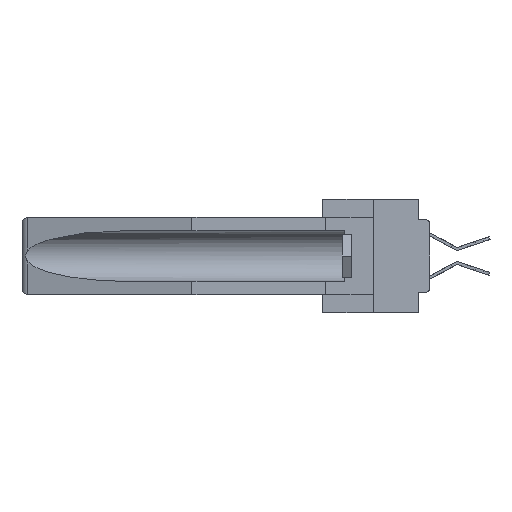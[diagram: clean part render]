
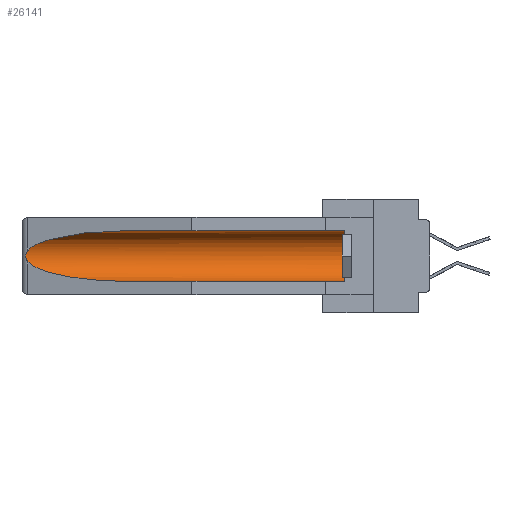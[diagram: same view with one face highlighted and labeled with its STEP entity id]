
A CAD part, left-side view. The second image highlights one B-rep face of the part: STEP entity #26141.
In plain terms, the highlighted cylindrical face has radius 2.857 mm (diameter 5.715 mm), a partial arc.
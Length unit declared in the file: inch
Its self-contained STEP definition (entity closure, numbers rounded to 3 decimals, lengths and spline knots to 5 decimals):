
#2087 = EDGE_LOOP ( 'NONE', ( #5907, #36978, #5419, #32253, #24840, #16142 ) ) ;
#3208 = CARTESIAN_POINT ( 'NONE',  ( 0.155, 1.07973, -0.059 ) ) ;
#3532 = AXIS2_PLACEMENT_3D ( 'NONE', #27109, #9231, #17881 ) ;
#4815 =( BOUNDED_CURVE ( )  B_SPLINE_CURVE ( 3, ( #15616, #17780, #27006, #27587 ),
 .UNSPECIFIED., .F., .F. ) 
 B_SPLINE_CURVE_WITH_KNOTS ( ( 4, 4 ),
 ( 0.1948, 1.5708 ),
 .UNSPECIFIED. ) 
 CURVE ( )  GEOMETRIC_REPRESENTATION_ITEM ( )  RATIONAL_B_SPLINE_CURVE ( ( 1., 0.848, 0.848, 1. ) ) 
 REPRESENTATION_ITEM ( '' )  );
#5419 = ORIENTED_EDGE ( 'NONE', *, *, #8309, .T. ) ;
#5594 = EDGE_CURVE ( 'NONE', #26791, #5600, #10086, .T. ) ;
#5600 = VERTEX_POINT ( 'NONE', #36031 ) ;
#5656 = CARTESIAN_POINT ( 'NONE',  ( 0.26655, 1.53094, -0.18657 ) ) ;
#5907 = ORIENTED_EDGE ( 'NONE', *, *, #5594, .T. ) ;
#7216 = VECTOR ( 'NONE', #13653, 39.37008 ) ;
#7429 = B_SPLINE_CURVE_WITH_KNOTS ( 'NONE', 3,
 ( #32557, #29431, #37891, #14514, #26503, #23558, #7831, #5656, #17658, #14709 ),
 .UNSPECIFIED., .F., .F.,
 ( 4, 2, 2, 2, 4 ),
 ( 0., 0.00029, 0.00058, 0.00087, 0.00117 ),
 .UNSPECIFIED. ) ;
#7769 = CARTESIAN_POINT ( 'NONE',  ( 0.155, 0.126, -0.059 ) ) ;
#7831 = CARTESIAN_POINT ( 'NONE',  ( 0.2673, 1.53269, -0.17917 ) ) ;
#8309 = EDGE_CURVE ( 'NONE', #30241, #24768, #4815, .T. ) ;
#8331 = VERTEX_POINT ( 'NONE', #15031 ) ;
#9231 = DIRECTION ( 'NONE',  ( 0., -1., 0. ) ) ;
#9416 = CARTESIAN_POINT ( 'NONE',  ( 0.26537, 1.52718, -0.19328 ) ) ;
#10086 =( BOUNDED_CURVE ( )  B_SPLINE_CURVE ( 3, ( #12041, #15400, #24240, #36415 ),
 .UNSPECIFIED., .F., .F. ) 
 B_SPLINE_CURVE_WITH_KNOTS ( ( 4, 4 ),
 ( 4.71239, 6.08839 ),
 .UNSPECIFIED. ) 
 CURVE ( )  GEOMETRIC_REPRESENTATION_ITEM ( )  RATIONAL_B_SPLINE_CURVE ( ( 1., 0.848, 0.848, 1. ) ) 
 REPRESENTATION_ITEM ( '' )  );
#10469 = EDGE_CURVE ( 'NONE', #5600, #30241, #7429, .T. ) ;
#10887 = CARTESIAN_POINT ( 'NONE',  ( 0.155, -0.30754, -0.284 ) ) ;
#12041 = CARTESIAN_POINT ( 'NONE',  ( 0.155, 1.07973, -0.059 ) ) ;
#12515 = DIRECTION ( 'NONE',  ( 0., 0., 1. ) ) ;
#13653 = DIRECTION ( 'NONE',  ( 0., 1., 0. ) ) ;
#14514 = CARTESIAN_POINT ( 'NONE',  ( 0.2673, 1.5327, -0.16383 ) ) ;
#14709 = CARTESIAN_POINT ( 'NONE',  ( 0.26537, 1.52718, -0.19328 ) ) ;
#15031 = CARTESIAN_POINT ( 'NONE',  ( 0.155, 0.126, -0.284 ) ) ;
#15400 = CARTESIAN_POINT ( 'NONE',  ( 0.21114, 1.30732, -0.059 ) ) ;
#15616 = CARTESIAN_POINT ( 'NONE',  ( 0.26537, 1.52718, -0.19328 ) ) ;
#16083 = EDGE_CURVE ( 'NONE', #8331, #24768, #29150, .T. ) ;
#16142 = ORIENTED_EDGE ( 'NONE', *, *, #20110, .T. ) ;
#16235 = LINE ( 'NONE', #25461, #25665 ) ;
#17658 = CARTESIAN_POINT ( 'NONE',  ( 0.26597, 1.5296, -0.19026 ) ) ;
#17780 = CARTESIAN_POINT ( 'NONE',  ( 0.25451, 1.48313, -0.24835 ) ) ;
#17881 = DIRECTION ( 'NONE',  ( 0., 0., 1. ) ) ;
#18233 = CYLINDRICAL_SURFACE ( 'NONE', #36060, 0.1125 ) ;
#19580 = DIRECTION ( 'NONE',  ( 0., 1., 0. ) ) ;
#20110 = EDGE_CURVE ( 'NONE', #21517, #26791, #16235, .T. ) ;
#20983 = DIRECTION ( 'NONE',  ( 0., 1., 0. ) ) ;
#21517 = VERTEX_POINT ( 'NONE', #7769 ) ;
#21754 = FACE_OUTER_BOUND ( 'NONE', #2087, .T. ) ;
#22970 = CIRCLE ( 'NONE', #3532, 0.1125 ) ;
#23558 = CARTESIAN_POINT ( 'NONE',  ( 0.2675, 1.53308, -0.17534 ) ) ;
#24240 = CARTESIAN_POINT ( 'NONE',  ( 0.25451, 1.48313, -0.09465 ) ) ;
#24768 = VERTEX_POINT ( 'NONE', #37865 ) ;
#24840 = ORIENTED_EDGE ( 'NONE', *, *, #36163, .T. ) ;
#25461 = CARTESIAN_POINT ( 'NONE',  ( 0.155, -0.30754, -0.059 ) ) ;
#25665 = VECTOR ( 'NONE', #19580, 39.37008 ) ;
#26141 = ADVANCED_FACE ( 'NONE', ( #21754 ), #18233, .F. ) ;
#26503 = CARTESIAN_POINT ( 'NONE',  ( 0.2675, 1.53308, -0.16763 ) ) ;
#26791 = VERTEX_POINT ( 'NONE', #3208 ) ;
#27006 = CARTESIAN_POINT ( 'NONE',  ( 0.21114, 1.30732, -0.284 ) ) ;
#27109 = CARTESIAN_POINT ( 'NONE',  ( 0.155, 0.126, -0.1715 ) ) ;
#27587 = CARTESIAN_POINT ( 'NONE',  ( 0.155, 1.07973, -0.284 ) ) ;
#29150 = LINE ( 'NONE', #10887, #7216 ) ;
#29431 = CARTESIAN_POINT ( 'NONE',  ( 0.26597, 1.52961, -0.15275 ) ) ;
#30241 = VERTEX_POINT ( 'NONE', #9416 ) ;
#32253 = ORIENTED_EDGE ( 'NONE', *, *, #16083, .F. ) ;
#32557 = CARTESIAN_POINT ( 'NONE',  ( 0.26537, 1.52718, -0.14972 ) ) ;
#36031 = CARTESIAN_POINT ( 'NONE',  ( 0.26537, 1.52718, -0.14972 ) ) ;
#36060 = AXIS2_PLACEMENT_3D ( 'NONE', #36669, #20983, #12515 ) ;
#36163 = EDGE_CURVE ( 'NONE', #8331, #21517, #22970, .T. ) ;
#36415 = CARTESIAN_POINT ( 'NONE',  ( 0.26537, 1.52718, -0.14972 ) ) ;
#36669 = CARTESIAN_POINT ( 'NONE',  ( 0.155, -0.30754, -0.1715 ) ) ;
#36978 = ORIENTED_EDGE ( 'NONE', *, *, #10469, .T. ) ;
#37865 = CARTESIAN_POINT ( 'NONE',  ( 0.155, 1.07973, -0.284 ) ) ;
#37891 = CARTESIAN_POINT ( 'NONE',  ( 0.26654, 1.53092, -0.15636 ) ) ;
